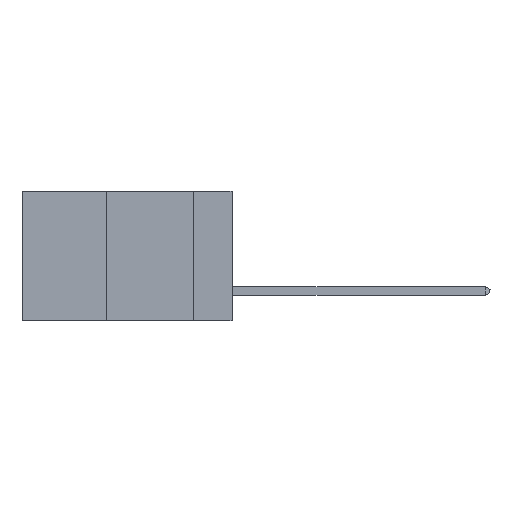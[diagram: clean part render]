
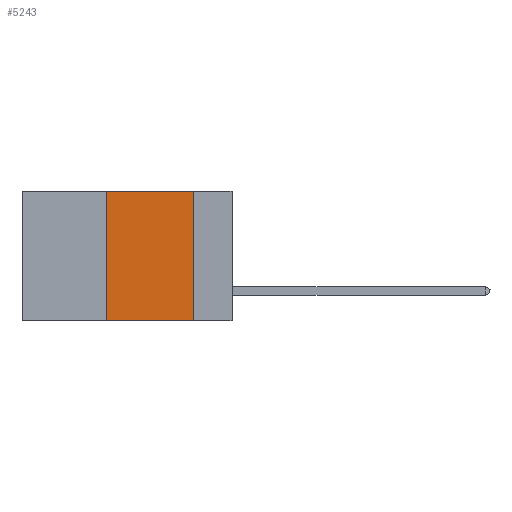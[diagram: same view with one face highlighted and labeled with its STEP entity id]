
A CAD part, left-side view. The second image highlights one B-rep face of the part: STEP entity #5243.
In plain terms, the highlighted planar face has unit normal (-1, 0, 0).
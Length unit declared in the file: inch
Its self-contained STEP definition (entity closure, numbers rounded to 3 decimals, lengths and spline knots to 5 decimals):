
#652 = CARTESIAN_POINT ( 'NONE',  ( 0., 0.6, -0.37 ) ) ;
#2730 = CARTESIAN_POINT ( 'NONE',  ( 0., 0.6, 0. ) ) ;
#5243 = ADVANCED_FACE ( 'NONE', ( #15600 ), #18554, .F. ) ;
#7676 = CARTESIAN_POINT ( 'NONE',  ( 0., 0.11, 0. ) ) ;
#9428 = AXIS2_PLACEMENT_3D ( 'NONE', #30231, #12060, #9694 ) ;
#9694 = DIRECTION ( 'NONE',  ( 0., 0., -1. ) ) ;
#9846 = EDGE_LOOP ( 'NONE', ( #29955, #10668, #38634, #32350 ) ) ;
#10664 = CARTESIAN_POINT ( 'NONE',  ( 0., 0.11, -0.37 ) ) ;
#10668 = ORIENTED_EDGE ( 'NONE', *, *, #34185, .F. ) ;
#12060 = DIRECTION ( 'NONE',  ( 1., 0., 0. ) ) ;
#13397 = LINE ( 'NONE', #22878, #35386 ) ;
#15099 = VERTEX_POINT ( 'NONE', #7676 ) ;
#15489 = CARTESIAN_POINT ( 'NONE',  ( 0., 0.36, -0.37 ) ) ;
#15600 = FACE_OUTER_BOUND ( 'NONE', #9846, .T. ) ;
#16494 = VERTEX_POINT ( 'NONE', #17727 ) ;
#17727 = CARTESIAN_POINT ( 'NONE',  ( 0., 0.36, 0. ) ) ;
#18189 = CARTESIAN_POINT ( 'NONE',  ( 0., 0.36, 0. ) ) ;
#18554 = PLANE ( 'NONE',  #9428 ) ;
#21299 = VECTOR ( 'NONE', #25114, 39.37008 ) ;
#21757 = LINE ( 'NONE', #652, #21299 ) ;
#21780 = EDGE_CURVE ( 'NONE', #15099, #33456, #13397, .T. ) ;
#22878 = CARTESIAN_POINT ( 'NONE',  ( 0., 0.11, 0. ) ) ;
#23044 = VECTOR ( 'NONE', #38824, 39.37008 ) ;
#24525 = DIRECTION ( 'NONE',  ( 0., 0., 1. ) ) ;
#25114 = DIRECTION ( 'NONE',  ( 0., -1., 0. ) ) ;
#25516 = EDGE_CURVE ( 'NONE', #36043, #16494, #27100, .T. ) ;
#27100 = LINE ( 'NONE', #18189, #28080 ) ;
#28080 = VECTOR ( 'NONE', #24525, 39.37008 ) ;
#29772 = LINE ( 'NONE', #2730, #23044 ) ;
#29955 = ORIENTED_EDGE ( 'NONE', *, *, #21780, .F. ) ;
#30231 = CARTESIAN_POINT ( 'NONE',  ( 0., 0.6, 0. ) ) ;
#32350 = ORIENTED_EDGE ( 'NONE', *, *, #36372, .T. ) ;
#33456 = VERTEX_POINT ( 'NONE', #10664 ) ;
#34185 = EDGE_CURVE ( 'NONE', #16494, #15099, #29772, .T. ) ;
#34905 = DIRECTION ( 'NONE',  ( 0., 0., -1. ) ) ;
#35386 = VECTOR ( 'NONE', #34905, 39.37008 ) ;
#36043 = VERTEX_POINT ( 'NONE', #15489 ) ;
#36372 = EDGE_CURVE ( 'NONE', #36043, #33456, #21757, .T. ) ;
#38634 = ORIENTED_EDGE ( 'NONE', *, *, #25516, .F. ) ;
#38824 = DIRECTION ( 'NONE',  ( 0., -1., 0. ) ) ;
